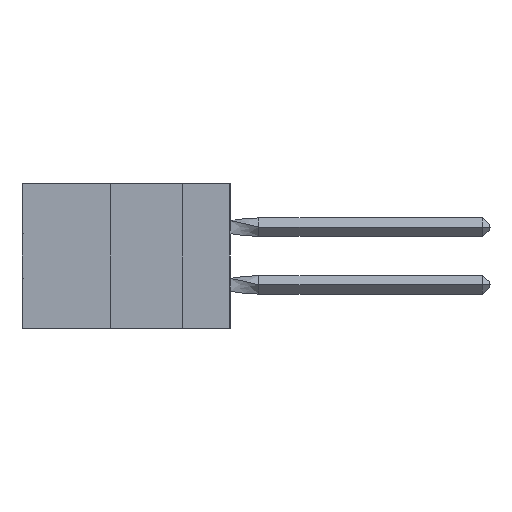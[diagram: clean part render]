
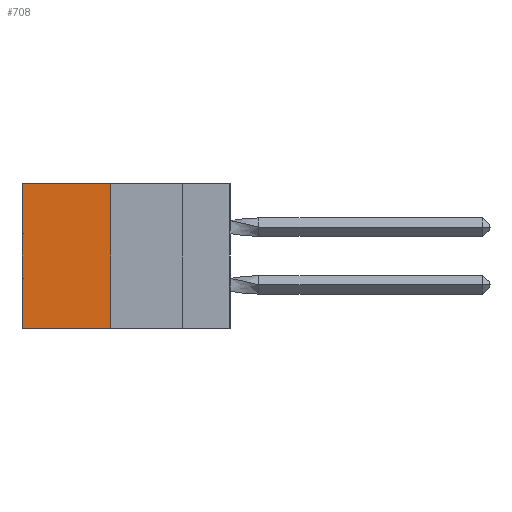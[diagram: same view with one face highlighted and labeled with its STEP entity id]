
A CAD part, left-side view. The second image highlights one B-rep face of the part: STEP entity #708.
In plain terms, the highlighted planar face has unit normal (-1, 0, 0).
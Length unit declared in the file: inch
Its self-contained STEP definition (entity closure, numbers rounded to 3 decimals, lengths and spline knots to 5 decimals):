
#126 = CARTESIAN_POINT ( 'NONE',  ( 0.305, 0.413, 0. ) ) ;
#637 = LINE ( 'NONE', #126, #16335 ) ;
#708 = ADVANCED_FACE ( 'NONE', ( #13074 ), #43053, .F. ) ;
#2236 = DIRECTION ( 'NONE',  ( 0., 0., -1. ) ) ;
#2561 = LINE ( 'NONE', #26128, #5256 ) ;
#5256 = VECTOR ( 'NONE', #43722, 39.37008 ) ;
#7169 = EDGE_LOOP ( 'NONE', ( #20950, #43613, #20211, #44055 ) ) ;
#7623 = CARTESIAN_POINT ( 'NONE',  ( 0.305, 0.72, 0. ) ) ;
#10650 = AXIS2_PLACEMENT_3D ( 'NONE', #26794, #32731, #29552 ) ;
#11341 = CARTESIAN_POINT ( 'NONE',  ( 0.305, 0.72, -0.5 ) ) ;
#13074 = FACE_OUTER_BOUND ( 'NONE', #7169, .T. ) ;
#13247 = EDGE_CURVE ( 'NONE', #38856, #24015, #637, .T. ) ;
#13771 = CARTESIAN_POINT ( 'NONE',  ( 0.305, 0.413, -0.5 ) ) ;
#16273 = CARTESIAN_POINT ( 'NONE',  ( 0.305, 0.413, -0.5 ) ) ;
#16335 = VECTOR ( 'NONE', #21344, 39.37008 ) ;
#18335 = DIRECTION ( 'NONE',  ( 0., 0., -1. ) ) ;
#20211 = ORIENTED_EDGE ( 'NONE', *, *, #20596, .F. ) ;
#20596 = EDGE_CURVE ( 'NONE', #38856, #36441, #32997, .T. ) ;
#20950 = ORIENTED_EDGE ( 'NONE', *, *, #37243, .T. ) ;
#21167 = LINE ( 'NONE', #11341, #34747 ) ;
#21344 = DIRECTION ( 'NONE',  ( 0., 1., 0. ) ) ;
#24015 = VERTEX_POINT ( 'NONE', #7623 ) ;
#25786 = EDGE_CURVE ( 'NONE', #36441, #30442, #2561, .T. ) ;
#26128 = CARTESIAN_POINT ( 'NONE',  ( 0.305, 0.413, -0.5 ) ) ;
#26794 = CARTESIAN_POINT ( 'NONE',  ( 0.305, 0.413, -0.5 ) ) ;
#28104 = VECTOR ( 'NONE', #2236, 39.37008 ) ;
#29552 = DIRECTION ( 'NONE',  ( 0., 0., -1. ) ) ;
#30442 = VERTEX_POINT ( 'NONE', #35017 ) ;
#32731 = DIRECTION ( 'NONE',  ( 1., 0., 0. ) ) ;
#32997 = LINE ( 'NONE', #16273, #28104 ) ;
#34747 = VECTOR ( 'NONE', #18335, 39.37008 ) ;
#35017 = CARTESIAN_POINT ( 'NONE',  ( 0.305, 0.72, -0.5 ) ) ;
#36441 = VERTEX_POINT ( 'NONE', #13771 ) ;
#37243 = EDGE_CURVE ( 'NONE', #24015, #30442, #21167, .T. ) ;
#38856 = VERTEX_POINT ( 'NONE', #41247 ) ;
#41247 = CARTESIAN_POINT ( 'NONE',  ( 0.305, 0.413, 0. ) ) ;
#43053 = PLANE ( 'NONE',  #10650 ) ;
#43613 = ORIENTED_EDGE ( 'NONE', *, *, #25786, .F. ) ;
#43722 = DIRECTION ( 'NONE',  ( 0., 1., 0. ) ) ;
#44055 = ORIENTED_EDGE ( 'NONE', *, *, #13247, .T. ) ;
